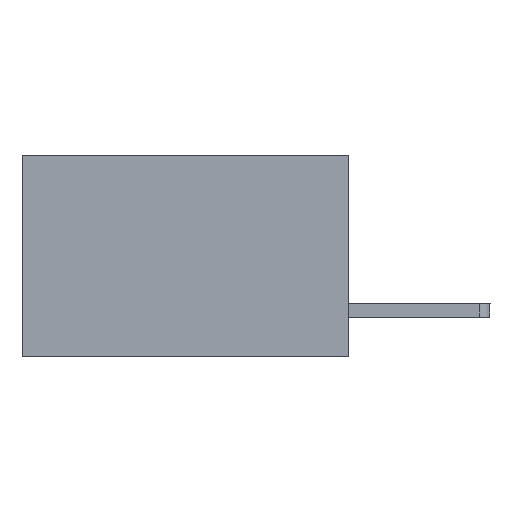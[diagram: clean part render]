
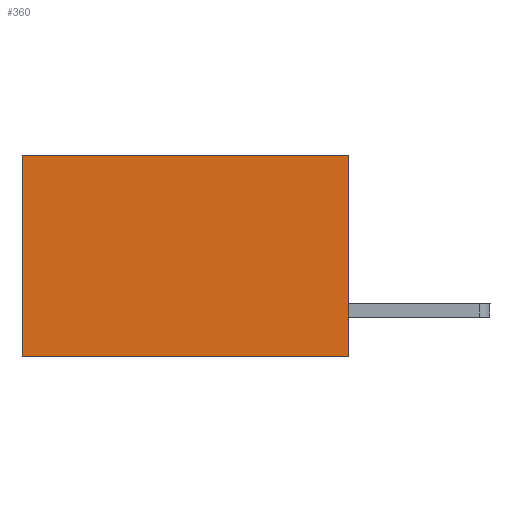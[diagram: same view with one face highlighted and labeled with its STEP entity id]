
A CAD part, left-side view. The second image highlights one B-rep face of the part: STEP entity #360.
In plain terms, the highlighted planar face has unit normal (-1, 0, 0).
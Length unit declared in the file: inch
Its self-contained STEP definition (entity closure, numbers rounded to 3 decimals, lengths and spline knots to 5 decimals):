
#54 = DIRECTION ( 'NONE',  ( 0., 0., -1. ) ) ;
#111 = VECTOR ( 'NONE', #54, 39.37008 ) ;
#360 = ADVANCED_FACE ( 'NONE', ( #12431 ), #12190, .F. ) ;
#614 = DIRECTION ( 'NONE',  ( 0., 1., 0. ) ) ;
#658 = VERTEX_POINT ( 'NONE', #1596 ) ;
#868 = VECTOR ( 'NONE', #2848, 39.37008 ) ;
#1199 = CARTESIAN_POINT ( 'NONE',  ( 0.298, 0.6, 0. ) ) ;
#1434 = DIRECTION ( 'NONE',  ( 0., 0., -1. ) ) ;
#1554 = EDGE_LOOP ( 'NONE', ( #7987, #6685, #9467, #12108 ) ) ;
#1596 = CARTESIAN_POINT ( 'NONE',  ( 0.298, 0.6, -0.37 ) ) ;
#2848 = DIRECTION ( 'NONE',  ( 0., 1., 0. ) ) ;
#3032 = CARTESIAN_POINT ( 'NONE',  ( 0.298, 0., 0. ) ) ;
#3573 = VERTEX_POINT ( 'NONE', #4216 ) ;
#3701 = CARTESIAN_POINT ( 'NONE',  ( 0.298, 0., 0. ) ) ;
#4216 = CARTESIAN_POINT ( 'NONE',  ( 0.298, 0., -0.37 ) ) ;
#5340 = CARTESIAN_POINT ( 'NONE',  ( 0.298, 0., -0.37 ) ) ;
#5750 = CARTESIAN_POINT ( 'NONE',  ( 0.298, 0., 0. ) ) ;
#6685 = ORIENTED_EDGE ( 'NONE', *, *, #9631, .F. ) ;
#6838 = LINE ( 'NONE', #3701, #868 ) ;
#7054 = VERTEX_POINT ( 'NONE', #3032 ) ;
#7528 = EDGE_CURVE ( 'NONE', #7054, #9805, #6838, .T. ) ;
#7923 = VECTOR ( 'NONE', #614, 39.37008 ) ;
#7987 = ORIENTED_EDGE ( 'NONE', *, *, #10111, .T. ) ;
#8335 = CARTESIAN_POINT ( 'NONE',  ( 0.298, 0., 0. ) ) ;
#8664 = VECTOR ( 'NONE', #1434, 39.37008 ) ;
#9305 = DIRECTION ( 'NONE',  ( 1., 0., 0. ) ) ;
#9467 = ORIENTED_EDGE ( 'NONE', *, *, #10356, .F. ) ;
#9583 = LINE ( 'NONE', #11909, #8664 ) ;
#9592 = LINE ( 'NONE', #5340, #7923 ) ;
#9631 = EDGE_CURVE ( 'NONE', #3573, #658, #9592, .T. ) ;
#9805 = VERTEX_POINT ( 'NONE', #1199 ) ;
#10111 = EDGE_CURVE ( 'NONE', #9805, #658, #9583, .T. ) ;
#10356 = EDGE_CURVE ( 'NONE', #7054, #3573, #11827, .T. ) ;
#10661 = AXIS2_PLACEMENT_3D ( 'NONE', #8335, #9305, #11241 ) ;
#11241 = DIRECTION ( 'NONE',  ( 0., 0., -1. ) ) ;
#11827 = LINE ( 'NONE', #5750, #111 ) ;
#11909 = CARTESIAN_POINT ( 'NONE',  ( 0.298, 0.6, 0. ) ) ;
#12108 = ORIENTED_EDGE ( 'NONE', *, *, #7528, .T. ) ;
#12190 = PLANE ( 'NONE',  #10661 ) ;
#12431 = FACE_OUTER_BOUND ( 'NONE', #1554, .T. ) ;
